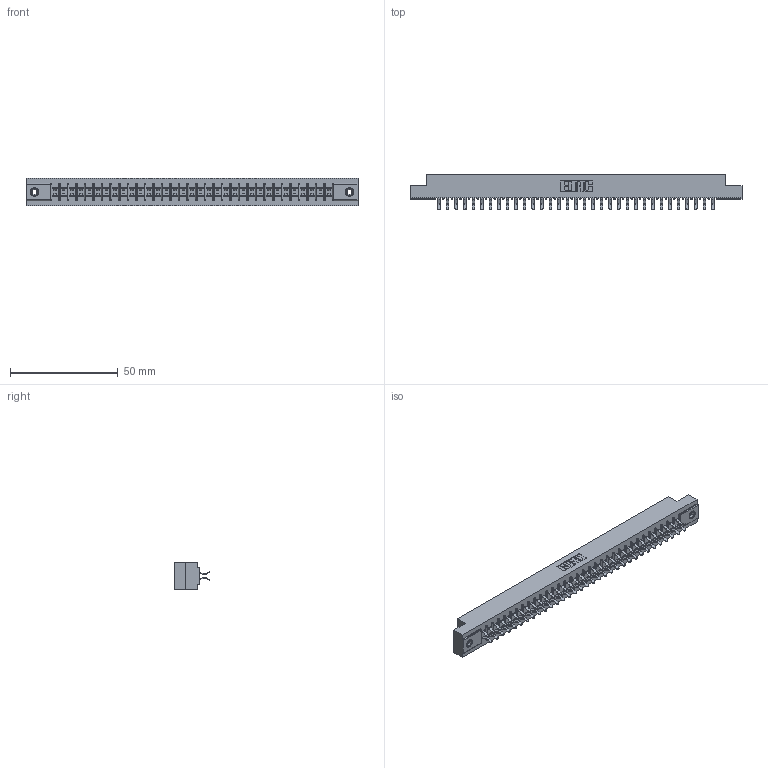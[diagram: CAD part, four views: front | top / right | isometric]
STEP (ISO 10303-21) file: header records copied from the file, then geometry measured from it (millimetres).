
FILE_DESCRIPTION (( 'STEP AP203' ), '1' );
FILE_NAME ('315-066-556-208.STEP', '2019-09-10T20:59:35', ( '' ), ( '' ), 'SwSTEP 2.0', 'SolidWorks 2016', '' );
FILE_SCHEMA (( 'CONFIG_CONTROL_DESIGN' ));
Length unit declared in the file: inch
Products named in the file (4): 345-250-001_345-250-003-102; 305-290-001_556; 315-066-556-208; 305 Part_.156 Dia
Assembly tree (69 placements, depth 2):
  315-066-556-208
    305 Part_.156 Dia
    305-290-001_556  x66
    345-250-001_345-250-003-102  x2
Bounding box: 153.77 x 16.64 x 12.7 mm (x, y, z)
Volume: 15974.7 mm3; surface area: 20152.2 mm2
Topology: 69 solids, 69 shells, 3872 faces, 11111 edges, 7222 vertices
Faces by surface type: plane 2146, cylinder 1578, sphere 132, cone 12, torus 4
Entity records: 38233 total; most frequent: CARTESIAN_POINT 6312, ORIENTED_EDGE 6258, DIRECTION 6127, EDGE_CURVE 3129, VECTOR 2513, LINE 2513, VERTEX_POINT 1992, AXIS2_PLACEMENT_3D 1807
